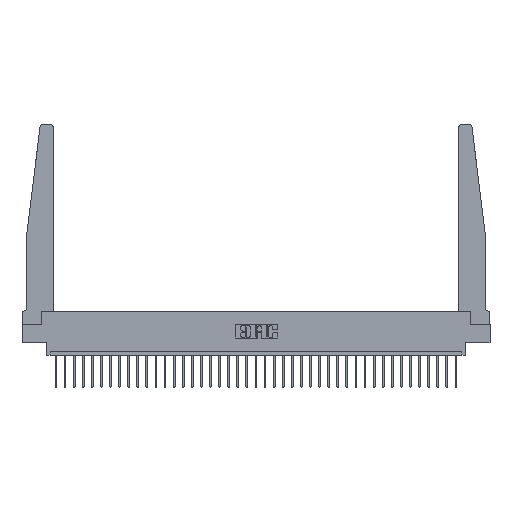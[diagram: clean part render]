
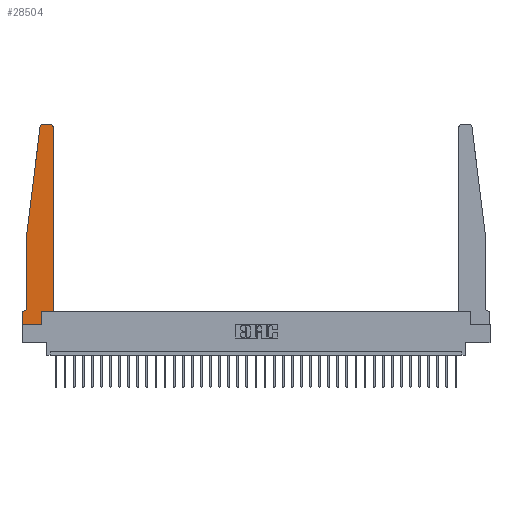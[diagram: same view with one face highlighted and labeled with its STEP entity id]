
A CAD part, top view. The second image highlights one B-rep face of the part: STEP entity #28504.
In plain terms, the highlighted planar face has unit normal (0, 0, 1).
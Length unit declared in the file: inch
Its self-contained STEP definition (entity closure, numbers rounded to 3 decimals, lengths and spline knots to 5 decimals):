
#292 = ORIENTED_EDGE ( 'NONE', *, *, #3776, .T. ) ;
#391 = CARTESIAN_POINT ( 'NONE',  ( 0.065, 0.2375, 0.37 ) ) ;
#464 = CARTESIAN_POINT ( 'NONE',  ( 0.065, 1.25, 0.37 ) ) ;
#1866 = CARTESIAN_POINT ( 'NONE',  ( 0.065, 1.25, 0.37 ) ) ;
#1990 = DIRECTION ( 'NONE',  ( -1., 0., 0. ) ) ;
#2004 = ORIENTED_EDGE ( 'NONE', *, *, #19090, .T. ) ;
#2253 = CARTESIAN_POINT ( 'NONE',  ( 0., 0., 0.37 ) ) ;
#2330 = LINE ( 'NONE', #27280, #16068 ) ;
#2589 = ORIENTED_EDGE ( 'NONE', *, *, #22924, .T. ) ;
#2701 = VERTEX_POINT ( 'NONE', #19878 ) ;
#3110 = DIRECTION ( 'NONE',  ( -0.122, -0.992, 0. ) ) ;
#3136 = CARTESIAN_POINT ( 'NONE',  ( 0.27653, 2.72, 0.37 ) ) ;
#3268 = LINE ( 'NONE', #464, #3860 ) ;
#3395 = ORIENTED_EDGE ( 'NONE', *, *, #5566, .T. ) ;
#3636 = ORIENTED_EDGE ( 'NONE', *, *, #19063, .T. ) ;
#3776 = EDGE_CURVE ( 'NONE', #24321, #5030, #16093, .T. ) ;
#3855 = VERTEX_POINT ( 'NONE', #21761 ) ;
#3859 = CARTESIAN_POINT ( 'NONE',  ( 0.065, 0.1875, 0.37 ) ) ;
#3860 = VECTOR ( 'NONE', #3110, 39.37008 ) ;
#4110 = CARTESIAN_POINT ( 'NONE',  ( 0., 0.1875, 0.37 ) ) ;
#4345 = VECTOR ( 'NONE', #29807, 39.37008 ) ;
#4491 = DIRECTION ( 'NONE',  ( 1., 0., 0. ) ) ;
#4746 = DIRECTION ( 'NONE',  ( 1., 0., 0. ) ) ;
#4838 = VERTEX_POINT ( 'NONE', #29946 ) ;
#4867 = VECTOR ( 'NONE', #14030, 39.37008 ) ;
#4912 = EDGE_CURVE ( 'NONE', #17613, #15311, #29367, .T. ) ;
#5030 = VERTEX_POINT ( 'NONE', #31089 ) ;
#5118 = CARTESIAN_POINT ( 'NONE',  ( 0.425, 0.18, 0.37 ) ) ;
#5566 = EDGE_CURVE ( 'NONE', #28077, #12075, #10915, .T. ) ;
#6013 = VECTOR ( 'NONE', #26038, 39.37008 ) ;
#6369 = ORIENTED_EDGE ( 'NONE', *, *, #19976, .T. ) ;
#6519 = CARTESIAN_POINT ( 'NONE',  ( 0.2605, 0.18, 0.37 ) ) ;
#7049 = CARTESIAN_POINT ( 'NONE',  ( 0.27653, 2.75, 0.37 ) ) ;
#8363 = EDGE_LOOP ( 'NONE', ( #23406, #292, #6369, #18064, #17587, #2589, #3395, #3636, #29006, #10924, #30182, #2004 ) ) ;
#8448 = VECTOR ( 'NONE', #27925, 39.37008 ) ;
#8588 = VECTOR ( 'NONE', #26628, 39.37008 ) ;
#8962 = AXIS2_PLACEMENT_3D ( 'NONE', #4110, #16928, #29729 ) ;
#9243 = DIRECTION ( 'NONE',  ( -1., 0., 0. ) ) ;
#9395 = DIRECTION ( 'NONE',  ( 1., 0., 0. ) ) ;
#10610 = CARTESIAN_POINT ( 'NONE',  ( 0., 0., 0.37 ) ) ;
#10915 = LINE ( 'NONE', #11074, #6013 ) ;
#10924 = ORIENTED_EDGE ( 'NONE', *, *, #32293, .T. ) ;
#11000 = EDGE_CURVE ( 'NONE', #2701, #24321, #21902, .T. ) ;
#11074 = CARTESIAN_POINT ( 'NONE',  ( 0., 0., 0.37 ) ) ;
#11606 = FACE_OUTER_BOUND ( 'NONE', #8363, .T. ) ;
#11692 = CARTESIAN_POINT ( 'NONE',  ( 0., 0.1875, 0.37 ) ) ;
#12075 = VERTEX_POINT ( 'NONE', #10610 ) ;
#12650 = DIRECTION ( 'NONE',  ( 0., 0., -1. ) ) ;
#13112 = LINE ( 'NONE', #5118, #8448 ) ;
#13294 = DIRECTION ( 'NONE',  ( 0., 0., 1. ) ) ;
#13797 = VECTOR ( 'NONE', #9243, 39.37008 ) ;
#14030 = DIRECTION ( 'NONE',  ( 0., 1., 0. ) ) ;
#14187 = LINE ( 'NONE', #6519, #4867 ) ;
#15311 = VERTEX_POINT ( 'NONE', #19440 ) ;
#16068 = VECTOR ( 'NONE', #4491, 39.37008 ) ;
#16093 = CIRCLE ( 'NONE', #31464, 0.03 ) ;
#16928 = DIRECTION ( 'NONE',  ( 0., 0., 1. ) ) ;
#17403 = CARTESIAN_POINT ( 'NONE',  ( 0.395, 2.72, 0.37 ) ) ;
#17487 = VECTOR ( 'NONE', #9395, 39.37008 ) ;
#17587 = ORIENTED_EDGE ( 'NONE', *, *, #4912, .T. ) ;
#17613 = VERTEX_POINT ( 'NONE', #391 ) ;
#18064 = ORIENTED_EDGE ( 'NONE', *, *, #31840, .T. ) ;
#18531 = CARTESIAN_POINT ( 'NONE',  ( 0.425, 2.72, 0.37 ) ) ;
#19063 = EDGE_CURVE ( 'NONE', #12075, #4838, #32043, .T. ) ;
#19090 = EDGE_CURVE ( 'NONE', #27974, #2701, #23823, .T. ) ;
#19093 = PLANE ( 'NONE',  #8962 ) ;
#19440 = CARTESIAN_POINT ( 'NONE',  ( 0.015, 0.1875, 0.37 ) ) ;
#19878 = CARTESIAN_POINT ( 'NONE',  ( 0.395, 2.75, 0.37 ) ) ;
#19916 = EDGE_CURVE ( 'NONE', #3855, #27974, #13112, .T. ) ;
#19976 = EDGE_CURVE ( 'NONE', #5030, #31246, #3268, .T. ) ;
#21761 = CARTESIAN_POINT ( 'NONE',  ( 0.425, 0.18, 0.37 ) ) ;
#21902 = LINE ( 'NONE', #32047, #13797 ) ;
#22924 = EDGE_CURVE ( 'NONE', #15311, #28077, #31972, .T. ) ;
#23406 = ORIENTED_EDGE ( 'NONE', *, *, #11000, .T. ) ;
#23431 = DIRECTION ( 'NONE',  ( 1., 0., 0. ) ) ;
#23823 = CIRCLE ( 'NONE', #30750, 0.03 ) ;
#24321 = VERTEX_POINT ( 'NONE', #7049 ) ;
#26038 = DIRECTION ( 'NONE',  ( 0., -1., 0. ) ) ;
#26628 = DIRECTION ( 'NONE',  ( -1., 0., 0. ) ) ;
#26785 = VERTEX_POINT ( 'NONE', #32431 ) ;
#27280 = CARTESIAN_POINT ( 'NONE',  ( 0.425, 0.18, 0.37 ) ) ;
#27535 = DIRECTION ( 'NONE',  ( 0., 0., 1. ) ) ;
#27925 = DIRECTION ( 'NONE',  ( 0., 1., 0. ) ) ;
#27974 = VERTEX_POINT ( 'NONE', #18531 ) ;
#28077 = VERTEX_POINT ( 'NONE', #11692 ) ;
#28504 = ADVANCED_FACE ( 'NONE', ( #11606 ), #19093, .T. ) ;
#29006 = ORIENTED_EDGE ( 'NONE', *, *, #31634, .T. ) ;
#29367 = CIRCLE ( 'NONE', #32032, 0.05 ) ;
#29729 = DIRECTION ( 'NONE',  ( 1., 0., 0. ) ) ;
#29773 = CARTESIAN_POINT ( 'NONE',  ( 0.015, 0.2375, 0.37 ) ) ;
#29807 = DIRECTION ( 'NONE',  ( 0., -1., 0. ) ) ;
#29946 = CARTESIAN_POINT ( 'NONE',  ( 0.2605, 0., 0.37 ) ) ;
#30182 = ORIENTED_EDGE ( 'NONE', *, *, #19916, .T. ) ;
#30750 = AXIS2_PLACEMENT_3D ( 'NONE', #17403, #27535, #4746 ) ;
#31076 = CARTESIAN_POINT ( 'NONE',  ( 0.065, 1.25, 0.37 ) ) ;
#31089 = CARTESIAN_POINT ( 'NONE',  ( 0.24675, 2.72367, 0.37 ) ) ;
#31246 = VERTEX_POINT ( 'NONE', #31076 ) ;
#31464 = AXIS2_PLACEMENT_3D ( 'NONE', #3136, #13294, #23431 ) ;
#31634 = EDGE_CURVE ( 'NONE', #4838, #26785, #14187, .T. ) ;
#31840 = EDGE_CURVE ( 'NONE', #31246, #17613, #32655, .T. ) ;
#31972 = LINE ( 'NONE', #3859, #8588 ) ;
#32032 = AXIS2_PLACEMENT_3D ( 'NONE', #29773, #12650, #1990 ) ;
#32043 = LINE ( 'NONE', #2253, #17487 ) ;
#32047 = CARTESIAN_POINT ( 'NONE',  ( 0.25, 2.75, 0.37 ) ) ;
#32293 = EDGE_CURVE ( 'NONE', #26785, #3855, #2330, .T. ) ;
#32431 = CARTESIAN_POINT ( 'NONE',  ( 0.2605, 0.18, 0.37 ) ) ;
#32655 = LINE ( 'NONE', #1866, #4345 ) ;
